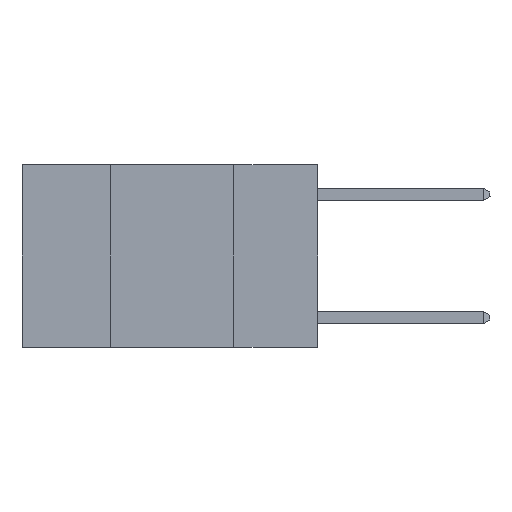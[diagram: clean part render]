
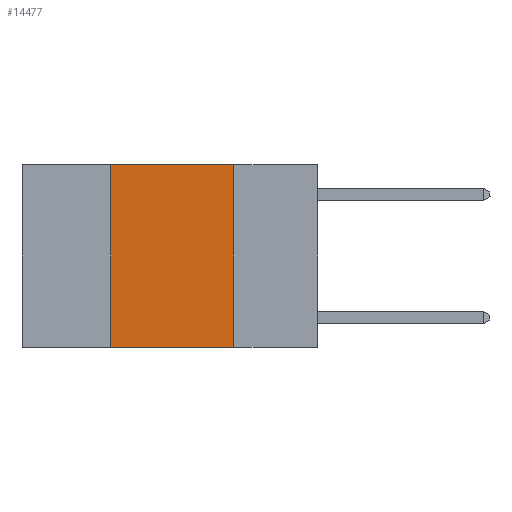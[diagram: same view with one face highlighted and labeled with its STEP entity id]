
A CAD part, left-side view. The second image highlights one B-rep face of the part: STEP entity #14477.
In plain terms, the highlighted planar face has unit normal (-1, 0, 0).
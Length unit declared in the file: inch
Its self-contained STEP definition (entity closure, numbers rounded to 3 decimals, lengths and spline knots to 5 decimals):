
#67 = LINE ( 'NONE', #8871, #14538 ) ;
#183 = VECTOR ( 'NONE', #4107, 39.37008 ) ;
#789 = DIRECTION ( 'NONE',  ( 1., 0., 0. ) ) ;
#877 = LINE ( 'NONE', #10416, #12751 ) ;
#911 = LINE ( 'NONE', #11015, #183 ) ;
#982 = EDGE_CURVE ( 'NONE', #8042, #10386, #877, .T. ) ;
#993 = FACE_OUTER_BOUND ( 'NONE', #10408, .T. ) ;
#1608 = ORIENTED_EDGE ( 'NONE', *, *, #982, .F. ) ;
#1930 = CARTESIAN_POINT ( 'NONE',  ( 0., 0.42, -0.37 ) ) ;
#3071 = CARTESIAN_POINT ( 'NONE',  ( 0., 0.6, 0. ) ) ;
#3574 = EDGE_CURVE ( 'NONE', #10021, #5452, #67, .T. ) ;
#4107 = DIRECTION ( 'NONE',  ( 0., -1., 0. ) ) ;
#4173 = AXIS2_PLACEMENT_3D ( 'NONE', #3071, #789, #8861 ) ;
#4331 = ORIENTED_EDGE ( 'NONE', *, *, #10626, .F. ) ;
#4534 = EDGE_CURVE ( 'NONE', #8042, #5452, #7998, .T. ) ;
#4687 = ORIENTED_EDGE ( 'NONE', *, *, #4534, .T. ) ;
#5452 = VERTEX_POINT ( 'NONE', #12574 ) ;
#7610 = VECTOR ( 'NONE', #12835, 39.37008 ) ;
#7998 = LINE ( 'NONE', #11739, #7610 ) ;
#8042 = VERTEX_POINT ( 'NONE', #1930 ) ;
#8141 = DIRECTION ( 'NONE',  ( 0., 0., 1. ) ) ;
#8320 = CARTESIAN_POINT ( 'NONE',  ( 0., 0.42, 0. ) ) ;
#8818 = PLANE ( 'NONE',  #4173 ) ;
#8861 = DIRECTION ( 'NONE',  ( 0., 0., -1. ) ) ;
#8871 = CARTESIAN_POINT ( 'NONE',  ( 0., 0.17, 0. ) ) ;
#10021 = VERTEX_POINT ( 'NONE', #13416 ) ;
#10081 = ORIENTED_EDGE ( 'NONE', *, *, #3574, .F. ) ;
#10386 = VERTEX_POINT ( 'NONE', #8320 ) ;
#10408 = EDGE_LOOP ( 'NONE', ( #10081, #4331, #1608, #4687 ) ) ;
#10416 = CARTESIAN_POINT ( 'NONE',  ( 0., 0.42, 0. ) ) ;
#10626 = EDGE_CURVE ( 'NONE', #10386, #10021, #911, .T. ) ;
#11015 = CARTESIAN_POINT ( 'NONE',  ( 0., 0.6, 0. ) ) ;
#11739 = CARTESIAN_POINT ( 'NONE',  ( 0., 0.6, -0.37 ) ) ;
#12334 = DIRECTION ( 'NONE',  ( 0., 0., -1. ) ) ;
#12574 = CARTESIAN_POINT ( 'NONE',  ( 0., 0.17, -0.37 ) ) ;
#12751 = VECTOR ( 'NONE', #8141, 39.37008 ) ;
#12835 = DIRECTION ( 'NONE',  ( 0., -1., 0. ) ) ;
#13416 = CARTESIAN_POINT ( 'NONE',  ( 0., 0.17, 0. ) ) ;
#14477 = ADVANCED_FACE ( 'NONE', ( #993 ), #8818, .F. ) ;
#14538 = VECTOR ( 'NONE', #12334, 39.37008 ) ;
